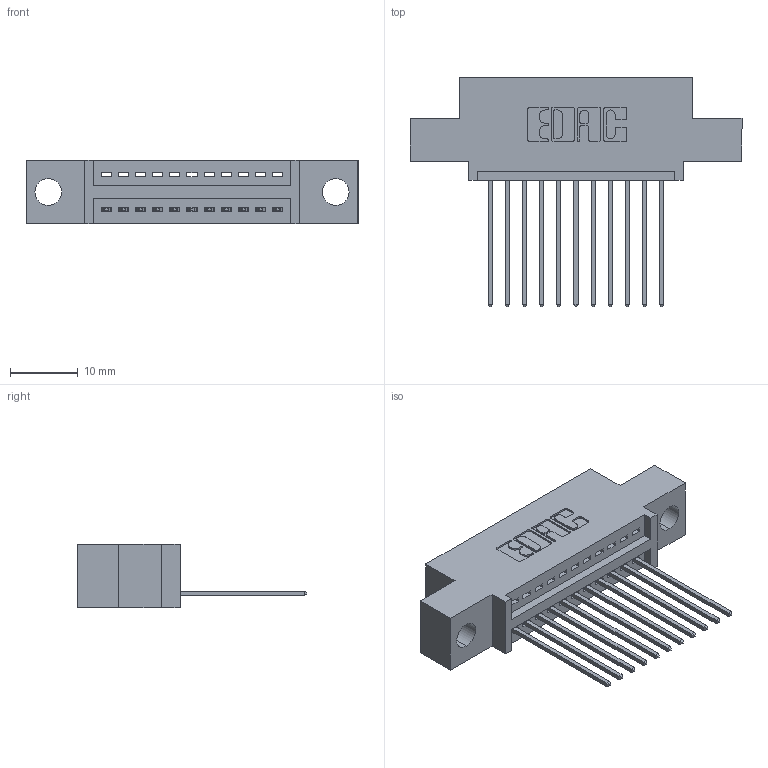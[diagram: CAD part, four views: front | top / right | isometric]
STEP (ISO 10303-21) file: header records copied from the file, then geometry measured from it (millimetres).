
FILE_DESCRIPTION (( 'STEP AP203' ), '1' );
FILE_NAME ('345-011-541-404.STEP', '2021-05-26T14:07:37', ( '' ), ( '' ), 'SwSTEP 2.0', 'SolidWorks 2020', '' );
FILE_SCHEMA (( 'CONFIG_CONTROL_DESIGN' ));
Length unit declared in the file: inch
Products named in the file (3): 345 Part_0.110 Offset - 0.156 Dia-TI; 345-011-541-404; 345-292-001_345-293-141
Assembly tree (12 placements, depth 2):
  345-011-541-404
    345 Part_0.110 Offset - 0.156 Dia-TI
    345-292-001_345-293-141  x11
Bounding box: 49.15 x 33.96 x 9.4 mm (x, y, z)
Volume: 4271.3 mm3; surface area: 5392.7 mm2
Topology: 12 solids, 12 shells, 782 faces, 2325 edges, 1534 vertices
Faces by surface type: plane 538, cylinder 244
Entity records: 13021 total; most frequent: CARTESIAN_POINT 2267, ORIENTED_EDGE 2210, DIRECTION 2023, EDGE_CURVE 1105, LINE 929, VECTOR 929, VERTEX_POINT 734, AXIS2_PLACEMENT_3D 547
